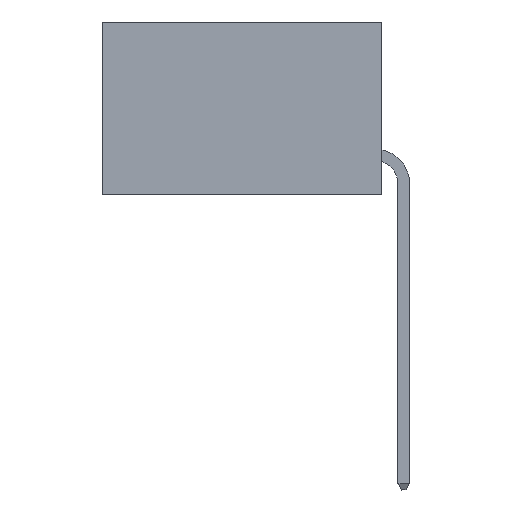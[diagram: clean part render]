
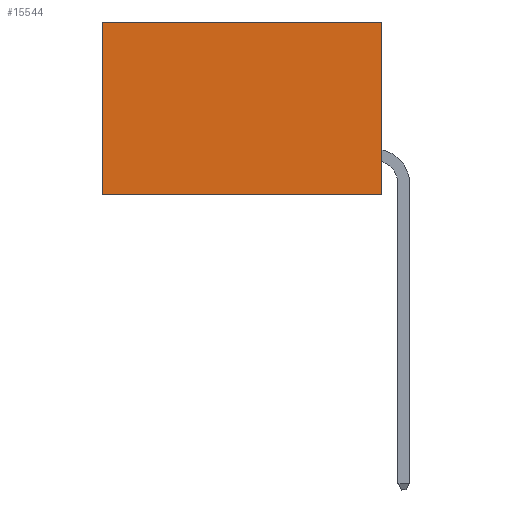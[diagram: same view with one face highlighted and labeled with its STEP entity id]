
A CAD part, left-side view. The second image highlights one B-rep face of the part: STEP entity #15544.
In plain terms, the highlighted planar face has unit normal (-1, 0, 0).
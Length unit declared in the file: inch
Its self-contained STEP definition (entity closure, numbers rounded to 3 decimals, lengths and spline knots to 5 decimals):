
#147 = CARTESIAN_POINT ( 'NONE',  ( 0.2875, 0., 0. ) ) ;
#689 = ORIENTED_EDGE ( 'NONE', *, *, #4337, .F. ) ;
#727 = ORIENTED_EDGE ( 'NONE', *, *, #14644, .T. ) ;
#894 = CARTESIAN_POINT ( 'NONE',  ( 0.2875, 0., 0. ) ) ;
#977 = CARTESIAN_POINT ( 'NONE',  ( 0.2875, 0.6, 0. ) ) ;
#1114 = DIRECTION ( 'NONE',  ( 0., 0., -1. ) ) ;
#1387 = VECTOR ( 'NONE', #16853, 39.37008 ) ;
#1510 = VECTOR ( 'NONE', #14272, 39.37008 ) ;
#2534 = EDGE_CURVE ( 'NONE', #5355, #17707, #4908, .T. ) ;
#2763 = FACE_OUTER_BOUND ( 'NONE', #5544, .T. ) ;
#3181 = VERTEX_POINT ( 'NONE', #11219 ) ;
#3252 = CARTESIAN_POINT ( 'NONE',  ( 0.2875, 0.6, 0. ) ) ;
#3807 = DIRECTION ( 'NONE',  ( 0., 0., -1. ) ) ;
#4337 = EDGE_CURVE ( 'NONE', #5355, #15671, #4856, .T. ) ;
#4856 = LINE ( 'NONE', #14893, #7814 ) ;
#4908 = LINE ( 'NONE', #147, #1510 ) ;
#5297 = EDGE_CURVE ( 'NONE', #15671, #3181, #9981, .T. ) ;
#5355 = VERTEX_POINT ( 'NONE', #894 ) ;
#5532 = DIRECTION ( 'NONE',  ( 0., 0., -1. ) ) ;
#5544 = EDGE_LOOP ( 'NONE', ( #727, #10847, #689, #7972 ) ) ;
#6980 = DIRECTION ( 'NONE',  ( 1., 0., 0. ) ) ;
#7814 = VECTOR ( 'NONE', #5532, 39.37008 ) ;
#7972 = ORIENTED_EDGE ( 'NONE', *, *, #2534, .T. ) ;
#9981 = LINE ( 'NONE', #16587, #1387 ) ;
#10245 = PLANE ( 'NONE',  #12688 ) ;
#10847 = ORIENTED_EDGE ( 'NONE', *, *, #5297, .F. ) ;
#11219 = CARTESIAN_POINT ( 'NONE',  ( 0.2875, 0.6, -0.37 ) ) ;
#11838 = CARTESIAN_POINT ( 'NONE',  ( 0.2875, 0., 0. ) ) ;
#12688 = AXIS2_PLACEMENT_3D ( 'NONE', #11838, #6980, #3807 ) ;
#14272 = DIRECTION ( 'NONE',  ( 0., 1., 0. ) ) ;
#14644 = EDGE_CURVE ( 'NONE', #17707, #3181, #15599, .T. ) ;
#14893 = CARTESIAN_POINT ( 'NONE',  ( 0.2875, 0., 0. ) ) ;
#15544 = ADVANCED_FACE ( 'NONE', ( #2763 ), #10245, .F. ) ;
#15599 = LINE ( 'NONE', #977, #19301 ) ;
#15671 = VERTEX_POINT ( 'NONE', #16678 ) ;
#16587 = CARTESIAN_POINT ( 'NONE',  ( 0.2875, 0., -0.37 ) ) ;
#16678 = CARTESIAN_POINT ( 'NONE',  ( 0.2875, 0., -0.37 ) ) ;
#16853 = DIRECTION ( 'NONE',  ( 0., 1., 0. ) ) ;
#17707 = VERTEX_POINT ( 'NONE', #3252 ) ;
#19301 = VECTOR ( 'NONE', #1114, 39.37008 ) ;
